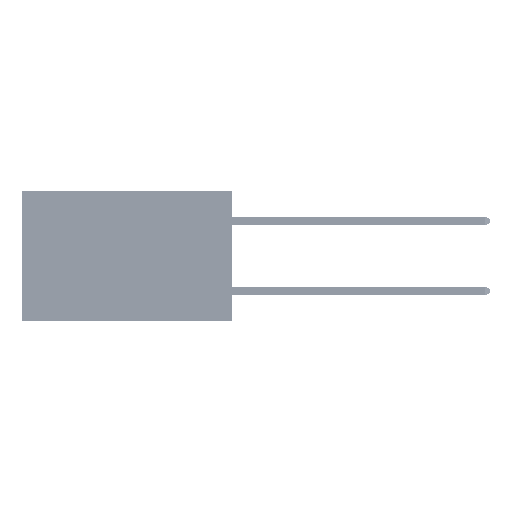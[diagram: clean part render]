
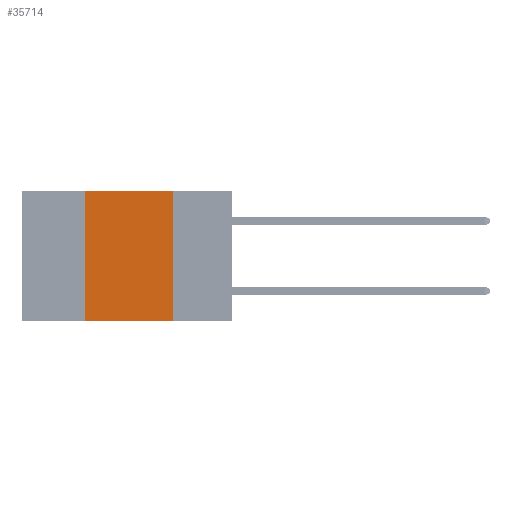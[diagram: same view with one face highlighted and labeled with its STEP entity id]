
A CAD part, left-side view. The second image highlights one B-rep face of the part: STEP entity #35714.
In plain terms, the highlighted planar face has unit normal (-1, 0, 0).
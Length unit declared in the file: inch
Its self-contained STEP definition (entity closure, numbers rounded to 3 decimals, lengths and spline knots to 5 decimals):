
#2353 = DIRECTION ( 'NONE',  ( 0., -1., 0. ) ) ;
#3569 = ORIENTED_EDGE ( 'NONE', *, *, #7866, .F. ) ;
#5209 = AXIS2_PLACEMENT_3D ( 'NONE', #34194, #18396, #10582 ) ;
#6949 = CARTESIAN_POINT ( 'NONE',  ( 0., 0.6, 0. ) ) ;
#7184 = LINE ( 'NONE', #44785, #22083 ) ;
#7866 = EDGE_CURVE ( 'NONE', #28373, #18220, #29658, .T. ) ;
#9711 = VERTEX_POINT ( 'NONE', #29880 ) ;
#10582 = DIRECTION ( 'NONE',  ( 0., 0., -1. ) ) ;
#14631 = LINE ( 'NONE', #25827, #48712 ) ;
#15426 = EDGE_CURVE ( 'NONE', #20892, #9711, #7184, .T. ) ;
#16185 = EDGE_CURVE ( 'NONE', #20892, #18220, #14631, .T. ) ;
#16754 = CARTESIAN_POINT ( 'NONE',  ( 0., 0.17, 0. ) ) ;
#16914 = DIRECTION ( 'NONE',  ( 0., 0., 1. ) ) ;
#18220 = VERTEX_POINT ( 'NONE', #40264 ) ;
#18396 = DIRECTION ( 'NONE',  ( 1., 0., 0. ) ) ;
#20892 = VERTEX_POINT ( 'NONE', #37835 ) ;
#22083 = VECTOR ( 'NONE', #16914, 39.37008 ) ;
#25827 = CARTESIAN_POINT ( 'NONE',  ( 0., 0.6, -0.37 ) ) ;
#28373 = VERTEX_POINT ( 'NONE', #50969 ) ;
#29658 = LINE ( 'NONE', #16754, #30883 ) ;
#29880 = CARTESIAN_POINT ( 'NONE',  ( 0., 0.42, 0. ) ) ;
#30883 = VECTOR ( 'NONE', #40497, 39.37008 ) ;
#31703 = ORIENTED_EDGE ( 'NONE', *, *, #16185, .T. ) ;
#33907 = ORIENTED_EDGE ( 'NONE', *, *, #15426, .F. ) ;
#34194 = CARTESIAN_POINT ( 'NONE',  ( 0., 0.6, 0. ) ) ;
#34731 = DIRECTION ( 'NONE',  ( 0., -1., 0. ) ) ;
#35714 = ADVANCED_FACE ( 'NONE', ( #50857 ), #50053, .F. ) ;
#37835 = CARTESIAN_POINT ( 'NONE',  ( 0., 0.42, -0.37 ) ) ;
#40264 = CARTESIAN_POINT ( 'NONE',  ( 0., 0.17, -0.37 ) ) ;
#40497 = DIRECTION ( 'NONE',  ( 0., 0., -1. ) ) ;
#41440 = LINE ( 'NONE', #6949, #50690 ) ;
#41869 = EDGE_LOOP ( 'NONE', ( #3569, #48539, #33907, #31703 ) ) ;
#44785 = CARTESIAN_POINT ( 'NONE',  ( 0., 0.42, 0. ) ) ;
#48539 = ORIENTED_EDGE ( 'NONE', *, *, #49107, .F. ) ;
#48712 = VECTOR ( 'NONE', #2353, 39.37008 ) ;
#49107 = EDGE_CURVE ( 'NONE', #9711, #28373, #41440, .T. ) ;
#50053 = PLANE ( 'NONE',  #5209 ) ;
#50690 = VECTOR ( 'NONE', #34731, 39.37008 ) ;
#50857 = FACE_OUTER_BOUND ( 'NONE', #41869, .T. ) ;
#50969 = CARTESIAN_POINT ( 'NONE',  ( 0., 0.17, 0. ) ) ;
